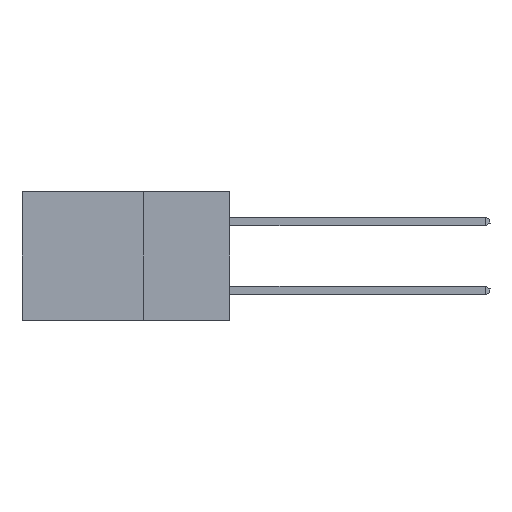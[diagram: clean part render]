
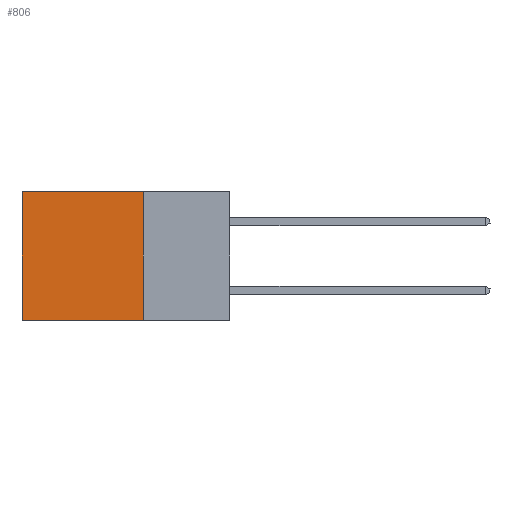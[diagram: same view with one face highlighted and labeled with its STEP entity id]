
A CAD part, left-side view. The second image highlights one B-rep face of the part: STEP entity #806.
In plain terms, the highlighted planar face has unit normal (-1, 0, 0).
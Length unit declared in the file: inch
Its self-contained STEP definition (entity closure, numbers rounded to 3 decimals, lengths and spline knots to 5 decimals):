
#138 = CARTESIAN_POINT ( 'NONE',  ( 0.298, 0.6, 0. ) ) ;
#366 = EDGE_CURVE ( 'NONE', #27503, #20265, #14678, .T. ) ;
#806 = ADVANCED_FACE ( 'NONE', ( #5339 ), #12692, .F. ) ;
#1269 = CARTESIAN_POINT ( 'NONE',  ( 0.298, 0.25, -0.37 ) ) ;
#1569 = CARTESIAN_POINT ( 'NONE',  ( 0.298, 0.6, 0. ) ) ;
#1931 = EDGE_LOOP ( 'NONE', ( #18850, #5574, #6813, #8548 ) ) ;
#2020 = DIRECTION ( 'NONE',  ( 0., 1., 0. ) ) ;
#2477 = DIRECTION ( 'NONE',  ( 0., 0., -1. ) ) ;
#3677 = VECTOR ( 'NONE', #6406, 39.37008 ) ;
#5110 = VERTEX_POINT ( 'NONE', #15662 ) ;
#5339 = FACE_OUTER_BOUND ( 'NONE', #1931, .T. ) ;
#5574 = ORIENTED_EDGE ( 'NONE', *, *, #13942, .F. ) ;
#6059 = CARTESIAN_POINT ( 'NONE',  ( 0.298, 0.25, 0. ) ) ;
#6406 = DIRECTION ( 'NONE',  ( 0., 0., -1. ) ) ;
#6813 = ORIENTED_EDGE ( 'NONE', *, *, #366, .F. ) ;
#7076 = EDGE_CURVE ( 'NONE', #27503, #28506, #10518, .T. ) ;
#8548 = ORIENTED_EDGE ( 'NONE', *, *, #7076, .T. ) ;
#9324 = LINE ( 'NONE', #1269, #10008 ) ;
#10008 = VECTOR ( 'NONE', #21006, 39.37008 ) ;
#10518 = LINE ( 'NONE', #6059, #21551 ) ;
#12692 = PLANE ( 'NONE',  #16233 ) ;
#13942 = EDGE_CURVE ( 'NONE', #20265, #5110, #9324, .T. ) ;
#14234 = CARTESIAN_POINT ( 'NONE',  ( 0.298, 0.25, 0. ) ) ;
#14678 = LINE ( 'NONE', #15177, #3677 ) ;
#14936 = VECTOR ( 'NONE', #2477, 39.37008 ) ;
#15177 = CARTESIAN_POINT ( 'NONE',  ( 0.298, 0.25, 0. ) ) ;
#15662 = CARTESIAN_POINT ( 'NONE',  ( 0.298, 0.6, -0.37 ) ) ;
#16233 = AXIS2_PLACEMENT_3D ( 'NONE', #28101, #21183, #16764 ) ;
#16764 = DIRECTION ( 'NONE',  ( 0., 0., -1. ) ) ;
#18490 = CARTESIAN_POINT ( 'NONE',  ( 0.298, 0.25, -0.37 ) ) ;
#18850 = ORIENTED_EDGE ( 'NONE', *, *, #27763, .T. ) ;
#20265 = VERTEX_POINT ( 'NONE', #18490 ) ;
#21006 = DIRECTION ( 'NONE',  ( 0., 1., 0. ) ) ;
#21183 = DIRECTION ( 'NONE',  ( 1., 0., 0. ) ) ;
#21551 = VECTOR ( 'NONE', #2020, 39.37008 ) ;
#24239 = LINE ( 'NONE', #138, #14936 ) ;
#27503 = VERTEX_POINT ( 'NONE', #14234 ) ;
#27763 = EDGE_CURVE ( 'NONE', #28506, #5110, #24239, .T. ) ;
#28101 = CARTESIAN_POINT ( 'NONE',  ( 0.298, 0.25, 0. ) ) ;
#28506 = VERTEX_POINT ( 'NONE', #1569 ) ;
